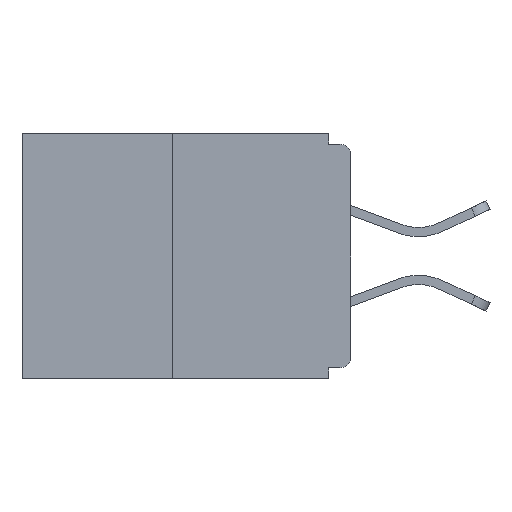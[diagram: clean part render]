
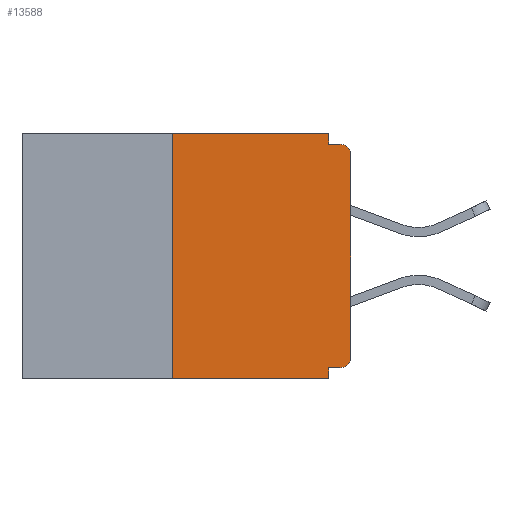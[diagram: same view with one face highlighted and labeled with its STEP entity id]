
A CAD part, left-side view. The second image highlights one B-rep face of the part: STEP entity #13588.
In plain terms, the highlighted planar face has unit normal (-1, 0, 0).
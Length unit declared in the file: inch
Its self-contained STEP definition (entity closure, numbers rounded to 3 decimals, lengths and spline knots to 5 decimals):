
#522 = AXIS2_PLACEMENT_3D ( 'NONE', #14666, #9115, #14449 ) ;
#951 = VECTOR ( 'NONE', #17949, 39.37008 ) ;
#1099 = LINE ( 'NONE', #13056, #13927 ) ;
#1128 = VERTEX_POINT ( 'NONE', #9824 ) ;
#1383 = LINE ( 'NONE', #9895, #11995 ) ;
#1718 = CARTESIAN_POINT ( 'NONE',  ( 0., 0.46, 0. ) ) ;
#2423 = CARTESIAN_POINT ( 'NONE',  ( 0., 0., 0. ) ) ;
#2917 = DIRECTION ( 'NONE',  ( 0., 0., 1. ) ) ;
#3407 = VERTEX_POINT ( 'NONE', #14835 ) ;
#3583 = CARTESIAN_POINT ( 'NONE',  ( 0., 0.015, -0.03 ) ) ;
#3796 = EDGE_CURVE ( 'NONE', #20515, #13274, #7274, .T. ) ;
#3873 = EDGE_CURVE ( 'NONE', #18574, #13274, #20473, .T. ) ;
#4249 = CARTESIAN_POINT ( 'NONE',  ( 0., 0.031, -0.015 ) ) ;
#5017 = VECTOR ( 'NONE', #20429, 39.37008 ) ;
#5092 = LINE ( 'NONE', #15158, #5017 ) ;
#5219 = CARTESIAN_POINT ( 'NONE',  ( 0., 0.031, -0.343 ) ) ;
#5566 = ORIENTED_EDGE ( 'NONE', *, *, #9162, .F. ) ;
#5998 = DIRECTION ( 'NONE',  ( 0., 0., 1. ) ) ;
#6141 = ORIENTED_EDGE ( 'NONE', *, *, #20815, .T. ) ;
#6149 = CARTESIAN_POINT ( 'NONE',  ( 0., 0.015, -0.328 ) ) ;
#6319 = ORIENTED_EDGE ( 'NONE', *, *, #10920, .T. ) ;
#6355 = DIRECTION ( 'NONE',  ( 0., 0., -1. ) ) ;
#6500 = DIRECTION ( 'NONE',  ( 0., 0., -1. ) ) ;
#6528 = FACE_OUTER_BOUND ( 'NONE', #12074, .T. ) ;
#6606 = VECTOR ( 'NONE', #8945, 39.37008 ) ;
#6765 = PLANE ( 'NONE',  #20941 ) ;
#7274 = CIRCLE ( 'NONE', #10828, 0.015 ) ;
#8213 = EDGE_CURVE ( 'NONE', #3407, #18574, #1099, .T. ) ;
#8385 = EDGE_CURVE ( 'NONE', #21531, #12871, #5092, .T. ) ;
#8642 = DIRECTION ( 'NONE',  ( -1., 0., 0. ) ) ;
#8945 = DIRECTION ( 'NONE',  ( 0., 0., -1. ) ) ;
#9115 = DIRECTION ( 'NONE',  ( -1., 0., 0. ) ) ;
#9162 = EDGE_CURVE ( 'NONE', #9481, #11401, #11217, .T. ) ;
#9481 = VERTEX_POINT ( 'NONE', #10871 ) ;
#9824 = CARTESIAN_POINT ( 'NONE',  ( 0., 0., -0.313 ) ) ;
#9873 = CARTESIAN_POINT ( 'NONE',  ( 0., 0.25, 0. ) ) ;
#9895 = CARTESIAN_POINT ( 'NONE',  ( 0., 0.46, 0. ) ) ;
#9951 = CARTESIAN_POINT ( 'NONE',  ( 0., 0.25, 0. ) ) ;
#10345 = EDGE_CURVE ( 'NONE', #12871, #19686, #20781, .T. ) ;
#10451 = ORIENTED_EDGE ( 'NONE', *, *, #8213, .F. ) ;
#10462 = EDGE_CURVE ( 'NONE', #1128, #20515, #21105, .T. ) ;
#10828 = AXIS2_PLACEMENT_3D ( 'NONE', #3583, #8642, #6500 ) ;
#10871 = CARTESIAN_POINT ( 'NONE',  ( 0., 0.25, -0.343 ) ) ;
#10920 = EDGE_CURVE ( 'NONE', #21531, #1128, #19458, .T. ) ;
#11117 = VECTOR ( 'NONE', #2917, 39.37008 ) ;
#11217 = LINE ( 'NONE', #9873, #11117 ) ;
#11356 = DIRECTION ( 'NONE',  ( 0., -1., 0. ) ) ;
#11401 = VERTEX_POINT ( 'NONE', #9951 ) ;
#11668 = CARTESIAN_POINT ( 'NONE',  ( 0., 0.031, -0.343 ) ) ;
#11982 = DIRECTION ( 'NONE',  ( 0., -1., 0. ) ) ;
#11995 = VECTOR ( 'NONE', #11356, 39.37008 ) ;
#12074 = EDGE_LOOP ( 'NONE', ( #13470, #5566, #6141, #20396, #21008, #6319, #20268, #20057, #12238, #10451 ) ) ;
#12238 = ORIENTED_EDGE ( 'NONE', *, *, #3873, .F. ) ;
#12294 = EDGE_CURVE ( 'NONE', #11401, #3407, #1383, .T. ) ;
#12300 = VECTOR ( 'NONE', #11982, 39.37008 ) ;
#12498 = CARTESIAN_POINT ( 'NONE',  ( 0., 0.015, -0.015 ) ) ;
#12871 = VERTEX_POINT ( 'NONE', #18378 ) ;
#12915 = CARTESIAN_POINT ( 'NONE',  ( 0., 0.46, -0.343 ) ) ;
#13056 = CARTESIAN_POINT ( 'NONE',  ( 0., 0.031, 0. ) ) ;
#13274 = VERTEX_POINT ( 'NONE', #12498 ) ;
#13338 = DIRECTION ( 'NONE',  ( 1., 0., 0. ) ) ;
#13470 = ORIENTED_EDGE ( 'NONE', *, *, #12294, .F. ) ;
#13588 = ADVANCED_FACE ( 'NONE', ( #6528 ), #6765, .F. ) ;
#13927 = VECTOR ( 'NONE', #6355, 39.37008 ) ;
#14449 = DIRECTION ( 'NONE',  ( 0., 0., -1. ) ) ;
#14666 = CARTESIAN_POINT ( 'NONE',  ( 0., 0.015, -0.313 ) ) ;
#14835 = CARTESIAN_POINT ( 'NONE',  ( 0., 0.031, 0. ) ) ;
#15158 = CARTESIAN_POINT ( 'NONE',  ( 0., 0., -0.328 ) ) ;
#15357 = DIRECTION ( 'NONE',  ( 0., 0., -1. ) ) ;
#15922 = VECTOR ( 'NONE', #5998, 39.37008 ) ;
#17949 = DIRECTION ( 'NONE',  ( 0., -1., 0. ) ) ;
#18378 = CARTESIAN_POINT ( 'NONE',  ( 0., 0.031, -0.328 ) ) ;
#18574 = VERTEX_POINT ( 'NONE', #4249 ) ;
#18623 = CARTESIAN_POINT ( 'NONE',  ( 0., 0., -0.03 ) ) ;
#19458 = CIRCLE ( 'NONE', #522, 0.015 ) ;
#19686 = VERTEX_POINT ( 'NONE', #11668 ) ;
#20057 = ORIENTED_EDGE ( 'NONE', *, *, #3796, .T. ) ;
#20141 = CARTESIAN_POINT ( 'NONE',  ( 0., 0., -0.015 ) ) ;
#20268 = ORIENTED_EDGE ( 'NONE', *, *, #10462, .T. ) ;
#20396 = ORIENTED_EDGE ( 'NONE', *, *, #10345, .F. ) ;
#20429 = DIRECTION ( 'NONE',  ( 0., 1., 0. ) ) ;
#20473 = LINE ( 'NONE', #20141, #12300 ) ;
#20515 = VERTEX_POINT ( 'NONE', #18623 ) ;
#20781 = LINE ( 'NONE', #5219, #6606 ) ;
#20815 = EDGE_CURVE ( 'NONE', #9481, #19686, #21090, .T. ) ;
#20941 = AXIS2_PLACEMENT_3D ( 'NONE', #1718, #13338, #15357 ) ;
#21008 = ORIENTED_EDGE ( 'NONE', *, *, #8385, .F. ) ;
#21090 = LINE ( 'NONE', #12915, #951 ) ;
#21105 = LINE ( 'NONE', #2423, #15922 ) ;
#21531 = VERTEX_POINT ( 'NONE', #6149 ) ;
